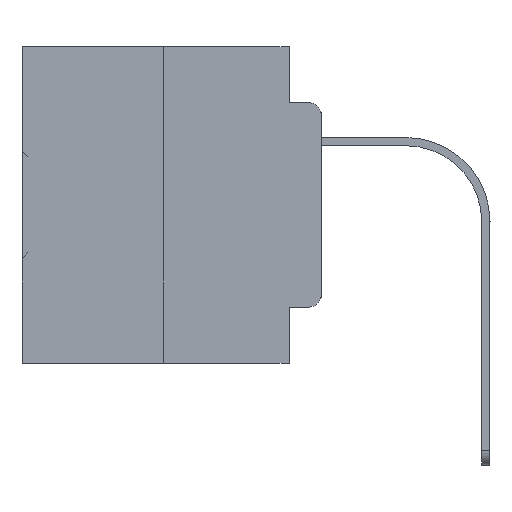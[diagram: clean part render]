
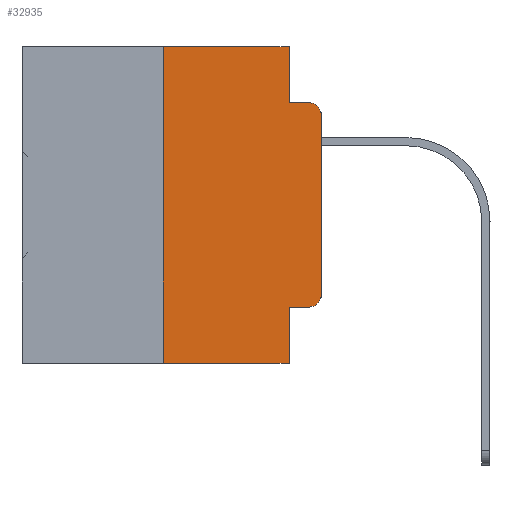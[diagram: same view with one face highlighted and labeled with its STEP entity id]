
A CAD part, left-side view. The second image highlights one B-rep face of the part: STEP entity #32935.
In plain terms, the highlighted planar face has unit normal (-1, 0, 0).
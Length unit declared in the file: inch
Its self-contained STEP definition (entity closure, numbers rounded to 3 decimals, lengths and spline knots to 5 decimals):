
#67 = VECTOR ( 'NONE', #21992, 39.37008 ) ;
#232 = DIRECTION ( 'NONE',  ( 0., 0., -1. ) ) ;
#372 = AXIS2_PLACEMENT_3D ( 'NONE', #31050, #25833, #16805 ) ;
#681 = EDGE_CURVE ( 'NONE', #29055, #7060, #16721, .T. ) ;
#1409 = EDGE_CURVE ( 'NONE', #2597, #34234, #15543, .T. ) ;
#2209 = CARTESIAN_POINT ( 'NONE',  ( 0., 0.25, -0.5 ) ) ;
#2491 = ORIENTED_EDGE ( 'NONE', *, *, #28759, .T. ) ;
#2597 = VERTEX_POINT ( 'NONE', #2209 ) ;
#2674 = DIRECTION ( 'NONE',  ( 0., -1., 0. ) ) ;
#3298 = CARTESIAN_POINT ( 'NONE',  ( 0., 0.02, -0.0885 ) ) ;
#3690 = EDGE_CURVE ( 'NONE', #35456, #29393, #36075, .T. ) ;
#3734 = VECTOR ( 'NONE', #9067, 39.37008 ) ;
#5274 = DIRECTION ( 'NONE',  ( 0., 0., 1. ) ) ;
#5719 = ORIENTED_EDGE ( 'NONE', *, *, #1409, .F. ) ;
#6737 = EDGE_CURVE ( 'NONE', #29055, #31201, #9625, .T. ) ;
#6804 = AXIS2_PLACEMENT_3D ( 'NONE', #23138, #19146, #232 ) ;
#7060 = VERTEX_POINT ( 'NONE', #8852 ) ;
#7327 = EDGE_CURVE ( 'NONE', #29393, #13207, #10675, .T. ) ;
#7971 = CARTESIAN_POINT ( 'NONE',  ( 0., 0.473, 0. ) ) ;
#8147 = FACE_OUTER_BOUND ( 'NONE', #23659, .T. ) ;
#8208 = CARTESIAN_POINT ( 'NONE',  ( 0., 0.051, -0.4115 ) ) ;
#8574 = DIRECTION ( 'NONE',  ( 0., -1., 0. ) ) ;
#8852 = CARTESIAN_POINT ( 'NONE',  ( 0., 0.02, -0.4115 ) ) ;
#9067 = DIRECTION ( 'NONE',  ( 0., -1., 0. ) ) ;
#9625 = LINE ( 'NONE', #34993, #13549 ) ;
#10675 = LINE ( 'NONE', #35681, #15348 ) ;
#13207 = VERTEX_POINT ( 'NONE', #3298 ) ;
#13549 = VECTOR ( 'NONE', #31831, 39.37008 ) ;
#13994 = EDGE_CURVE ( 'NONE', #34234, #35456, #25757, .T. ) ;
#14849 = VECTOR ( 'NONE', #30152, 39.37008 ) ;
#15348 = VECTOR ( 'NONE', #24175, 39.37008 ) ;
#15501 = ORIENTED_EDGE ( 'NONE', *, *, #26000, .T. ) ;
#15543 = LINE ( 'NONE', #26820, #14849 ) ;
#16721 = LINE ( 'NONE', #27824, #24802 ) ;
#16805 = DIRECTION ( 'NONE',  ( 0., 0., -1. ) ) ;
#16896 = ORIENTED_EDGE ( 'NONE', *, *, #27436, .T. ) ;
#17047 = CARTESIAN_POINT ( 'NONE',  ( 0., 0., -0.1085 ) ) ;
#17231 = EDGE_CURVE ( 'NONE', #2597, #31201, #31284, .T. ) ;
#17591 = ORIENTED_EDGE ( 'NONE', *, *, #681, .T. ) ;
#18636 = CARTESIAN_POINT ( 'NONE',  ( 0., 0.051, 0. ) ) ;
#19146 = DIRECTION ( 'NONE',  ( -1., 0., 0. ) ) ;
#19271 = VECTOR ( 'NONE', #5274, 39.37008 ) ;
#19753 = ORIENTED_EDGE ( 'NONE', *, *, #7327, .F. ) ;
#19913 = CARTESIAN_POINT ( 'NONE',  ( 0., 0., -0.3915 ) ) ;
#20987 = CIRCLE ( 'NONE', #6804, 0.02 ) ;
#21273 = VERTEX_POINT ( 'NONE', #17047 ) ;
#21654 = DIRECTION ( 'NONE',  ( 1., 0., 0. ) ) ;
#21992 = DIRECTION ( 'NONE',  ( 0., 0., -1. ) ) ;
#22206 = VERTEX_POINT ( 'NONE', #19913 ) ;
#23138 = CARTESIAN_POINT ( 'NONE',  ( 0., 0.02, -0.1085 ) ) ;
#23659 = EDGE_LOOP ( 'NONE', ( #16896, #15501, #19753, #34073, #27419, #5719, #32816, #26852, #17591, #2491 ) ) ;
#24076 = CARTESIAN_POINT ( 'NONE',  ( 0., 0.051, -0.0885 ) ) ;
#24175 = DIRECTION ( 'NONE',  ( 0., -1., 0. ) ) ;
#24802 = VECTOR ( 'NONE', #2674, 39.37008 ) ;
#25757 = LINE ( 'NONE', #25931, #33039 ) ;
#25833 = DIRECTION ( 'NONE',  ( -1., 0., 0. ) ) ;
#25931 = CARTESIAN_POINT ( 'NONE',  ( 0., 0.473, 0. ) ) ;
#26000 = EDGE_CURVE ( 'NONE', #21273, #13207, #20987, .T. ) ;
#26318 = CARTESIAN_POINT ( 'NONE',  ( 0., 0.051, -0.5 ) ) ;
#26820 = CARTESIAN_POINT ( 'NONE',  ( 0., 0.25, 0. ) ) ;
#26852 = ORIENTED_EDGE ( 'NONE', *, *, #6737, .F. ) ;
#27391 = DIRECTION ( 'NONE',  ( 0., 0., -1. ) ) ;
#27419 = ORIENTED_EDGE ( 'NONE', *, *, #13994, .F. ) ;
#27436 = EDGE_CURVE ( 'NONE', #22206, #21273, #30998, .T. ) ;
#27824 = CARTESIAN_POINT ( 'NONE',  ( 0., 0.051, -0.4115 ) ) ;
#28759 = EDGE_CURVE ( 'NONE', #7060, #22206, #32266, .T. ) ;
#29055 = VERTEX_POINT ( 'NONE', #8208 ) ;
#29393 = VERTEX_POINT ( 'NONE', #24076 ) ;
#30147 = CARTESIAN_POINT ( 'NONE',  ( 0., 0.051, 0. ) ) ;
#30152 = DIRECTION ( 'NONE',  ( 0., 0., 1. ) ) ;
#30629 = CARTESIAN_POINT ( 'NONE',  ( 0., 0., 0. ) ) ;
#30998 = LINE ( 'NONE', #30629, #19271 ) ;
#31050 = CARTESIAN_POINT ( 'NONE',  ( 0., 0.02, -0.3915 ) ) ;
#31201 = VERTEX_POINT ( 'NONE', #26318 ) ;
#31284 = LINE ( 'NONE', #34428, #3734 ) ;
#31831 = DIRECTION ( 'NONE',  ( 0., 0., -1. ) ) ;
#32266 = CIRCLE ( 'NONE', #372, 0.02 ) ;
#32816 = ORIENTED_EDGE ( 'NONE', *, *, #17231, .T. ) ;
#32935 = ADVANCED_FACE ( 'NONE', ( #8147 ), #33322, .F. ) ;
#33039 = VECTOR ( 'NONE', #8574, 39.37008 ) ;
#33207 = AXIS2_PLACEMENT_3D ( 'NONE', #7971, #21654, #27391 ) ;
#33322 = PLANE ( 'NONE',  #33207 ) ;
#34073 = ORIENTED_EDGE ( 'NONE', *, *, #3690, .F. ) ;
#34234 = VERTEX_POINT ( 'NONE', #36109 ) ;
#34428 = CARTESIAN_POINT ( 'NONE',  ( 0., 0.473, -0.5 ) ) ;
#34993 = CARTESIAN_POINT ( 'NONE',  ( 0., 0.051, 0. ) ) ;
#35456 = VERTEX_POINT ( 'NONE', #18636 ) ;
#35681 = CARTESIAN_POINT ( 'NONE',  ( 0., 0.051, -0.0885 ) ) ;
#36075 = LINE ( 'NONE', #30147, #67 ) ;
#36109 = CARTESIAN_POINT ( 'NONE',  ( 0., 0.25, 0. ) ) ;
